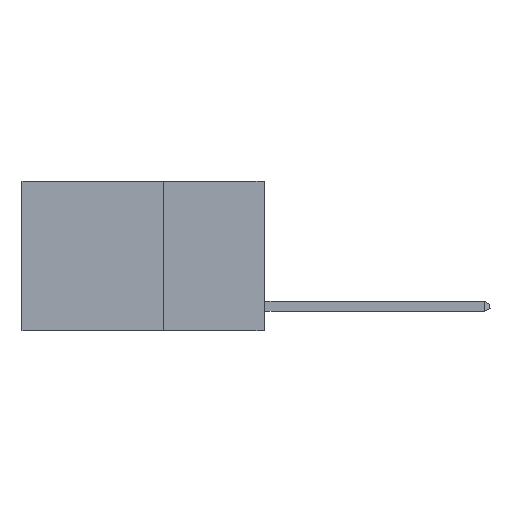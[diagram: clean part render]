
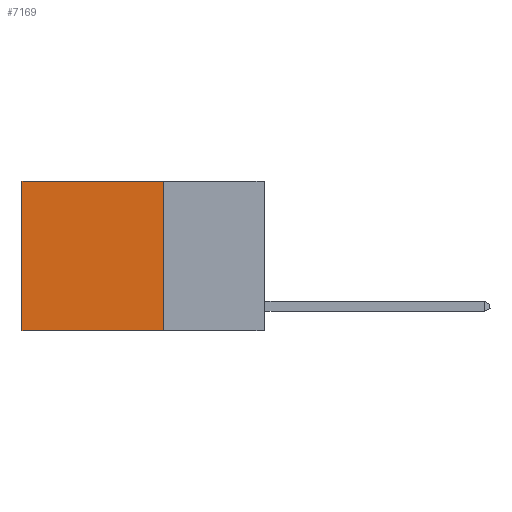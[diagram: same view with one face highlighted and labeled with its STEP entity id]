
A CAD part, left-side view. The second image highlights one B-rep face of the part: STEP entity #7169.
In plain terms, the highlighted planar face has unit normal (-1, 0, 0).
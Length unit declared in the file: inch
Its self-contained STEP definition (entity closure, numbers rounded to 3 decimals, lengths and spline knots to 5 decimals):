
#310 = CARTESIAN_POINT ( 'NONE',  ( 0.2625, 0.25, 0. ) ) ;
#562 = FACE_OUTER_BOUND ( 'NONE', #7917, .T. ) ;
#750 = ORIENTED_EDGE ( 'NONE', *, *, #1381, .F. ) ;
#1381 = EDGE_CURVE ( 'NONE', #2808, #2402, #2130, .T. ) ;
#1631 = LINE ( 'NONE', #9437, #11987 ) ;
#1669 = DIRECTION ( 'NONE',  ( 0., 0., -1. ) ) ;
#1887 = CARTESIAN_POINT ( 'NONE',  ( 0.2625, 0.25, 0. ) ) ;
#2130 = LINE ( 'NONE', #310, #8980 ) ;
#2257 = ORIENTED_EDGE ( 'NONE', *, *, #5701, .T. ) ;
#2402 = VERTEX_POINT ( 'NONE', #9049 ) ;
#2808 = VERTEX_POINT ( 'NONE', #1887 ) ;
#3200 = VECTOR ( 'NONE', #9689, 39.37008 ) ;
#3328 = ORIENTED_EDGE ( 'NONE', *, *, #8589, .F. ) ;
#4265 = VECTOR ( 'NONE', #5842, 39.37008 ) ;
#4384 = EDGE_CURVE ( 'NONE', #12112, #8566, #1631, .T. ) ;
#4531 = PLANE ( 'NONE',  #7619 ) ;
#5530 = DIRECTION ( 'NONE',  ( 0., 0., -1. ) ) ;
#5666 = LINE ( 'NONE', #6518, #3200 ) ;
#5701 = EDGE_CURVE ( 'NONE', #2808, #12112, #5666, .T. ) ;
#5842 = DIRECTION ( 'NONE',  ( 0., 1., 0. ) ) ;
#6118 = DIRECTION ( 'NONE',  ( 0., 0., -1. ) ) ;
#6518 = CARTESIAN_POINT ( 'NONE',  ( 0.2625, 0.25, 0. ) ) ;
#6620 = CARTESIAN_POINT ( 'NONE',  ( 0.2625, 0.25, -0.37 ) ) ;
#7169 = ADVANCED_FACE ( 'NONE', ( #562 ), #4531, .F. ) ;
#7615 = CARTESIAN_POINT ( 'NONE',  ( 0.2625, 0.6, -0.37 ) ) ;
#7619 = AXIS2_PLACEMENT_3D ( 'NONE', #8543, #12830, #1669 ) ;
#7676 = LINE ( 'NONE', #6620, #4265 ) ;
#7917 = EDGE_LOOP ( 'NONE', ( #9845, #3328, #750, #2257 ) ) ;
#8543 = CARTESIAN_POINT ( 'NONE',  ( 0.2625, 0.25, 0. ) ) ;
#8566 = VERTEX_POINT ( 'NONE', #7615 ) ;
#8589 = EDGE_CURVE ( 'NONE', #2402, #8566, #7676, .T. ) ;
#8980 = VECTOR ( 'NONE', #6118, 39.37008 ) ;
#9049 = CARTESIAN_POINT ( 'NONE',  ( 0.2625, 0.25, -0.37 ) ) ;
#9437 = CARTESIAN_POINT ( 'NONE',  ( 0.2625, 0.6, 0. ) ) ;
#9689 = DIRECTION ( 'NONE',  ( 0., 1., 0. ) ) ;
#9845 = ORIENTED_EDGE ( 'NONE', *, *, #4384, .T. ) ;
#10117 = CARTESIAN_POINT ( 'NONE',  ( 0.2625, 0.6, 0. ) ) ;
#11987 = VECTOR ( 'NONE', #5530, 39.37008 ) ;
#12112 = VERTEX_POINT ( 'NONE', #10117 ) ;
#12830 = DIRECTION ( 'NONE',  ( 1., 0., 0. ) ) ;
